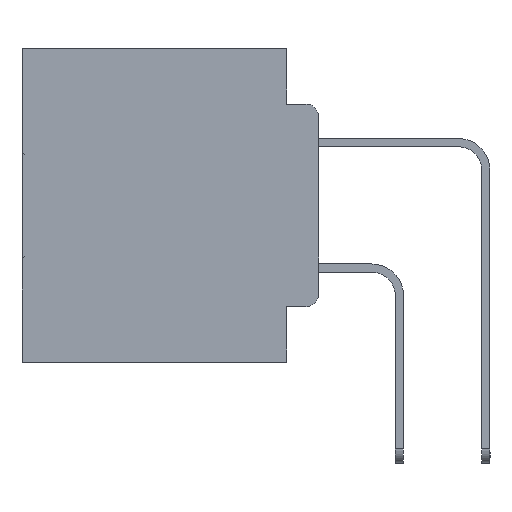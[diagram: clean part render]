
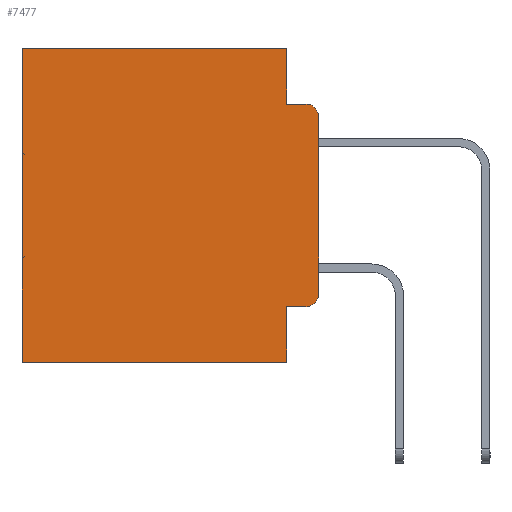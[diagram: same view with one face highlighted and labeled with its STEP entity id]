
A CAD part, left-side view. The second image highlights one B-rep face of the part: STEP entity #7477.
In plain terms, the highlighted planar face has unit normal (-1, 0, 0).
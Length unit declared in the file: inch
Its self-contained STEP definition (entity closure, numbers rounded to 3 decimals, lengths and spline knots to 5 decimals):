
#170 = VERTEX_POINT ( 'NONE', #27064 ) ;
#245 = ORIENTED_EDGE ( 'NONE', *, *, #9602, .F. ) ;
#773 = DIRECTION ( 'NONE',  ( -1., 0., 0. ) ) ;
#937 = CARTESIAN_POINT ( 'NONE',  ( 0.298, 0.02, -0.3915 ) ) ;
#1236 = EDGE_CURVE ( 'NONE', #14525, #11279, #18763, .T. ) ;
#1735 = CARTESIAN_POINT ( 'NONE',  ( 0.298, 0.02, -0.0885 ) ) ;
#2024 = FACE_OUTER_BOUND ( 'NONE', #11922, .T. ) ;
#2027 = VECTOR ( 'NONE', #25517, 39.37008 ) ;
#2133 = ORIENTED_EDGE ( 'NONE', *, *, #13376, .F. ) ;
#2724 = ORIENTED_EDGE ( 'NONE', *, *, #23866, .F. ) ;
#3655 = VERTEX_POINT ( 'NONE', #25362 ) ;
#4561 = AXIS2_PLACEMENT_3D ( 'NONE', #22645, #19560, #33300 ) ;
#4708 = LINE ( 'NONE', #15180, #19721 ) ;
#4996 = VERTEX_POINT ( 'NONE', #10863 ) ;
#5694 = DIRECTION ( 'NONE',  ( 0., 1., 0. ) ) ;
#5885 = CIRCLE ( 'NONE', #28936, 0.02 ) ;
#6803 = VECTOR ( 'NONE', #17474, 39.37008 ) ;
#7169 = ORIENTED_EDGE ( 'NONE', *, *, #1236, .T. ) ;
#7477 = ADVANCED_FACE ( 'NONE', ( #2024 ), #30043, .F. ) ;
#7644 = AXIS2_PLACEMENT_3D ( 'NONE', #937, #773, #23498 ) ;
#9602 = EDGE_CURVE ( 'NONE', #3655, #29055, #10739, .T. ) ;
#9871 = LINE ( 'NONE', #30522, #19652 ) ;
#10259 = VECTOR ( 'NONE', #22196, 39.37008 ) ;
#10739 = LINE ( 'NONE', #31736, #31635 ) ;
#10863 = CARTESIAN_POINT ( 'NONE',  ( 0.298, 0.473, -0.5 ) ) ;
#11279 = VERTEX_POINT ( 'NONE', #31018 ) ;
#11922 = EDGE_LOOP ( 'NONE', ( #2724, #16744, #2133, #18855, #7169, #21015, #32256, #245, #22978, #12660 ) ) ;
#12070 = VERTEX_POINT ( 'NONE', #1735 ) ;
#12660 = ORIENTED_EDGE ( 'NONE', *, *, #32601, .T. ) ;
#12708 = EDGE_CURVE ( 'NONE', #14525, #25413, #30852, .T. ) ;
#12974 = DIRECTION ( 'NONE',  ( -1., 0., 0. ) ) ;
#13313 = CARTESIAN_POINT ( 'NONE',  ( 0.298, 0.051, 0. ) ) ;
#13376 = EDGE_CURVE ( 'NONE', #25413, #12070, #19610, .T. ) ;
#14217 = LINE ( 'NONE', #14545, #6803 ) ;
#14525 = VERTEX_POINT ( 'NONE', #13313 ) ;
#14545 = CARTESIAN_POINT ( 'NONE',  ( 0.298, 0., 0. ) ) ;
#15180 = CARTESIAN_POINT ( 'NONE',  ( 0.298, 0., -0.5 ) ) ;
#15694 = EDGE_CURVE ( 'NONE', #3655, #170, #9871, .T. ) ;
#16744 = ORIENTED_EDGE ( 'NONE', *, *, #28410, .T. ) ;
#17435 = DIRECTION ( 'NONE',  ( 0., 0., -1. ) ) ;
#17474 = DIRECTION ( 'NONE',  ( 0., 0., -1. ) ) ;
#17976 = CARTESIAN_POINT ( 'NONE',  ( 0.298, 0.02, -0.1085 ) ) ;
#18501 = CARTESIAN_POINT ( 'NONE',  ( 0.298, 0., -0.3915 ) ) ;
#18687 = VERTEX_POINT ( 'NONE', #18501 ) ;
#18763 = LINE ( 'NONE', #29256, #27054 ) ;
#18855 = ORIENTED_EDGE ( 'NONE', *, *, #12708, .F. ) ;
#19560 = DIRECTION ( 'NONE',  ( 1., 0., 0. ) ) ;
#19610 = LINE ( 'NONE', #32687, #10259 ) ;
#19652 = VECTOR ( 'NONE', #25878, 39.37008 ) ;
#19721 = VECTOR ( 'NONE', #25670, 39.37008 ) ;
#21015 = ORIENTED_EDGE ( 'NONE', *, *, #30938, .T. ) ;
#22196 = DIRECTION ( 'NONE',  ( 0., -1., 0. ) ) ;
#22645 = CARTESIAN_POINT ( 'NONE',  ( 0.298, 0., 0. ) ) ;
#22978 = ORIENTED_EDGE ( 'NONE', *, *, #15694, .T. ) ;
#23310 = DIRECTION ( 'NONE',  ( 0., 0., -1. ) ) ;
#23488 = DIRECTION ( 'NONE',  ( 0., 0., -1. ) ) ;
#23498 = DIRECTION ( 'NONE',  ( 0., 0., -1. ) ) ;
#23589 = VECTOR ( 'NONE', #17435, 39.37008 ) ;
#23866 = EDGE_CURVE ( 'NONE', #32092, #18687, #14217, .T. ) ;
#24832 = LINE ( 'NONE', #27903, #23589 ) ;
#25362 = CARTESIAN_POINT ( 'NONE',  ( 0.298, 0.051, -0.4115 ) ) ;
#25413 = VERTEX_POINT ( 'NONE', #30717 ) ;
#25517 = DIRECTION ( 'NONE',  ( 0., 0., -1. ) ) ;
#25670 = DIRECTION ( 'NONE',  ( 0., 1., 0. ) ) ;
#25756 = CIRCLE ( 'NONE', #7644, 0.02 ) ;
#25878 = DIRECTION ( 'NONE',  ( 0., -1., 0. ) ) ;
#26102 = CARTESIAN_POINT ( 'NONE',  ( 0.298, 0., -0.1085 ) ) ;
#27054 = VECTOR ( 'NONE', #5694, 39.37008 ) ;
#27064 = CARTESIAN_POINT ( 'NONE',  ( 0.298, 0.02, -0.4115 ) ) ;
#27184 = CARTESIAN_POINT ( 'NONE',  ( 0.298, 0.051, -0.5 ) ) ;
#27903 = CARTESIAN_POINT ( 'NONE',  ( 0.298, 0.473, 0. ) ) ;
#28098 = CARTESIAN_POINT ( 'NONE',  ( 0.298, 0.051, 0. ) ) ;
#28410 = EDGE_CURVE ( 'NONE', #32092, #12070, #5885, .T. ) ;
#28936 = AXIS2_PLACEMENT_3D ( 'NONE', #17976, #12974, #23310 ) ;
#29055 = VERTEX_POINT ( 'NONE', #27184 ) ;
#29256 = CARTESIAN_POINT ( 'NONE',  ( 0.298, 0., 0. ) ) ;
#30043 = PLANE ( 'NONE',  #4561 ) ;
#30522 = CARTESIAN_POINT ( 'NONE',  ( 0.298, 0.051, -0.4115 ) ) ;
#30717 = CARTESIAN_POINT ( 'NONE',  ( 0.298, 0.051, -0.0885 ) ) ;
#30852 = LINE ( 'NONE', #28098, #2027 ) ;
#30938 = EDGE_CURVE ( 'NONE', #11279, #4996, #24832, .T. ) ;
#31018 = CARTESIAN_POINT ( 'NONE',  ( 0.298, 0.473, 0. ) ) ;
#31188 = EDGE_CURVE ( 'NONE', #29055, #4996, #4708, .T. ) ;
#31635 = VECTOR ( 'NONE', #23488, 39.37008 ) ;
#31736 = CARTESIAN_POINT ( 'NONE',  ( 0.298, 0.051, 0. ) ) ;
#32092 = VERTEX_POINT ( 'NONE', #26102 ) ;
#32256 = ORIENTED_EDGE ( 'NONE', *, *, #31188, .F. ) ;
#32601 = EDGE_CURVE ( 'NONE', #170, #18687, #25756, .T. ) ;
#32687 = CARTESIAN_POINT ( 'NONE',  ( 0.298, 0.051, -0.0885 ) ) ;
#33300 = DIRECTION ( 'NONE',  ( 0., 0., -1. ) ) ;
